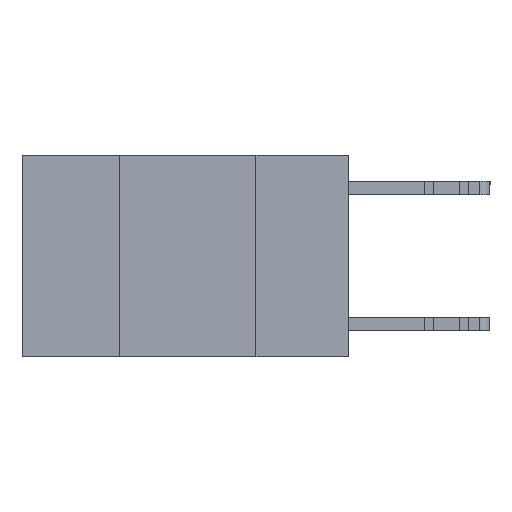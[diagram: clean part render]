
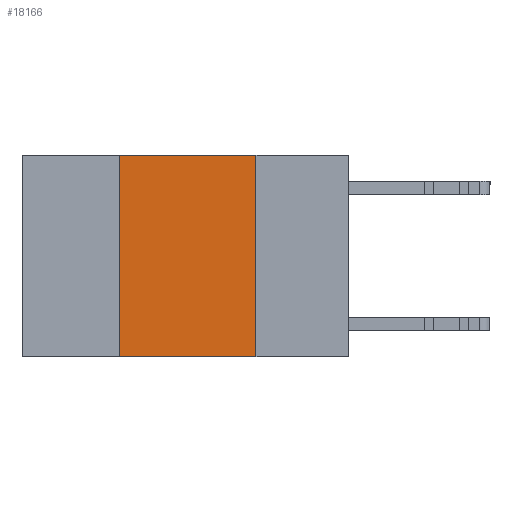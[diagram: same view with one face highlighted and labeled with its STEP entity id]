
A CAD part, left-side view. The second image highlights one B-rep face of the part: STEP entity #18166.
In plain terms, the highlighted planar face has unit normal (-1, 0, 0).
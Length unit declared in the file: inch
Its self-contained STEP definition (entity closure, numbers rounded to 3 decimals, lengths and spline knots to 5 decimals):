
#602 = DIRECTION ( 'NONE',  ( 0., 0., 1. ) ) ;
#2841 = ORIENTED_EDGE ( 'NONE', *, *, #27853, .F. ) ;
#3478 = DIRECTION ( 'NONE',  ( 0., -1., 0. ) ) ;
#4032 = ORIENTED_EDGE ( 'NONE', *, *, #4040, .T. ) ;
#4040 = EDGE_CURVE ( 'NONE', #23013, #24328, #7951, .T. ) ;
#4430 = LINE ( 'NONE', #6812, #24890 ) ;
#4870 = DIRECTION ( 'NONE',  ( 0., 0., -1. ) ) ;
#6086 = CARTESIAN_POINT ( 'NONE',  ( 0., 0.6, 0. ) ) ;
#6417 = ORIENTED_EDGE ( 'NONE', *, *, #14091, .F. ) ;
#6812 = CARTESIAN_POINT ( 'NONE',  ( 0., 0.17, 0. ) ) ;
#7951 = LINE ( 'NONE', #17073, #25507 ) ;
#8998 = CARTESIAN_POINT ( 'NONE',  ( 0., 0.17, 0. ) ) ;
#9259 = LINE ( 'NONE', #9571, #11909 ) ;
#9410 = EDGE_LOOP ( 'NONE', ( #6417, #12282, #2841, #4032 ) ) ;
#9571 = CARTESIAN_POINT ( 'NONE',  ( 0., 0.42, 0. ) ) ;
#11909 = VECTOR ( 'NONE', #602, 39.37008 ) ;
#12282 = ORIENTED_EDGE ( 'NONE', *, *, #26317, .F. ) ;
#14091 = EDGE_CURVE ( 'NONE', #24000, #24328, #4430, .T. ) ;
#14501 = DIRECTION ( 'NONE',  ( 0., 0., -1. ) ) ;
#15512 = CARTESIAN_POINT ( 'NONE',  ( 0., 0.6, 0. ) ) ;
#17073 = CARTESIAN_POINT ( 'NONE',  ( 0., 0.6, -0.37 ) ) ;
#17908 = LINE ( 'NONE', #15512, #21913 ) ;
#18166 = ADVANCED_FACE ( 'NONE', ( #25924 ), #23529, .F. ) ;
#19258 = AXIS2_PLACEMENT_3D ( 'NONE', #6086, #28506, #14501 ) ;
#21913 = VECTOR ( 'NONE', #24682, 39.37008 ) ;
#23013 = VERTEX_POINT ( 'NONE', #26923 ) ;
#23370 = VERTEX_POINT ( 'NONE', #23897 ) ;
#23529 = PLANE ( 'NONE',  #19258 ) ;
#23897 = CARTESIAN_POINT ( 'NONE',  ( 0., 0.42, 0. ) ) ;
#24000 = VERTEX_POINT ( 'NONE', #8998 ) ;
#24328 = VERTEX_POINT ( 'NONE', #28468 ) ;
#24682 = DIRECTION ( 'NONE',  ( 0., -1., 0. ) ) ;
#24890 = VECTOR ( 'NONE', #4870, 39.37008 ) ;
#25507 = VECTOR ( 'NONE', #3478, 39.37008 ) ;
#25924 = FACE_OUTER_BOUND ( 'NONE', #9410, .T. ) ;
#26317 = EDGE_CURVE ( 'NONE', #23370, #24000, #17908, .T. ) ;
#26923 = CARTESIAN_POINT ( 'NONE',  ( 0., 0.42, -0.37 ) ) ;
#27853 = EDGE_CURVE ( 'NONE', #23013, #23370, #9259, .T. ) ;
#28468 = CARTESIAN_POINT ( 'NONE',  ( 0., 0.17, -0.37 ) ) ;
#28506 = DIRECTION ( 'NONE',  ( 1., 0., 0. ) ) ;
